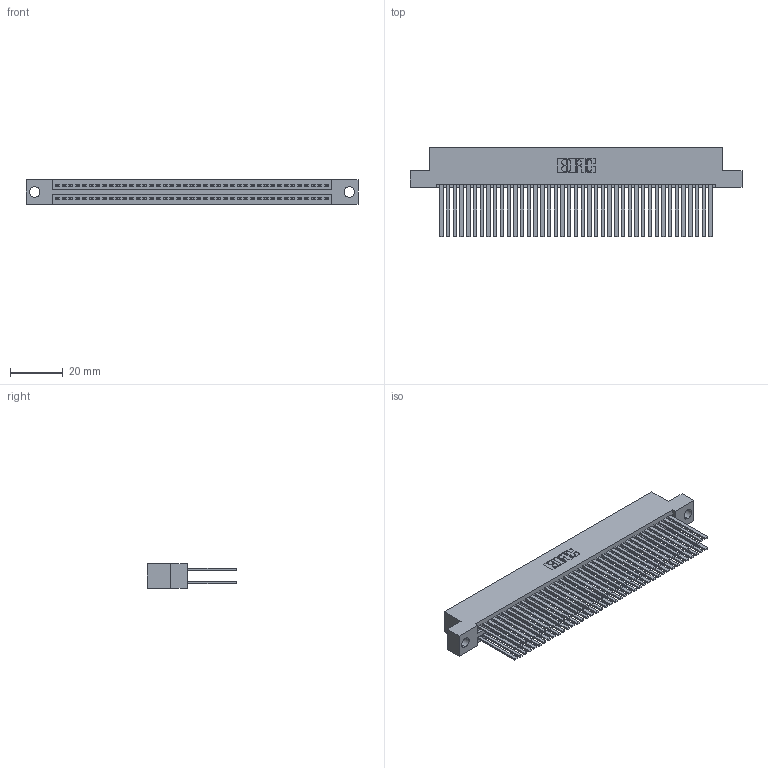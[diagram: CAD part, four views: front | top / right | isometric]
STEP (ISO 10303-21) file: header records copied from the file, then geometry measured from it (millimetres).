
FILE_DESCRIPTION (( 'STEP AP203' ), '1' );
FILE_NAME ('345-082-544-204.STEP', '2018-10-03T22:38:34', ( '' ), ( '' ), 'SwSTEP 2.0', 'SolidWorks 2016', '' );
FILE_SCHEMA (( 'CONFIG_CONTROL_DESIGN' ));
Length unit declared in the file: inch
Products named in the file (3): 345-292-001_345-293-144; 345-082-544-204; 345 Part_Flush Mounting Lugs - 0.156 Dia-TH
Assembly tree (83 placements, depth 2):
  345-082-544-204
    345 Part_Flush Mounting Lugs - 0.156 Dia-TH
    345-292-001_345-293-144  x82
Bounding box: 125.35 x 33.96 x 9.4 mm (x, y, z)
Volume: 13228.9 mm3; surface area: 22719.4 mm2
Topology: 83 solids, 83 shells, 3734 faces, 11083 edges, 7278 vertices
Faces by surface type: plane 2458, cylinder 1276
Entity records: 32123 total; most frequent: CARTESIAN_POINT 5384, ORIENTED_EDGE 5318, DIRECTION 4747, EDGE_CURVE 2659, LINE 2367, VECTOR 2367, VERTEX_POINT 1770, AXIS2_PLACEMENT_3D 1190
